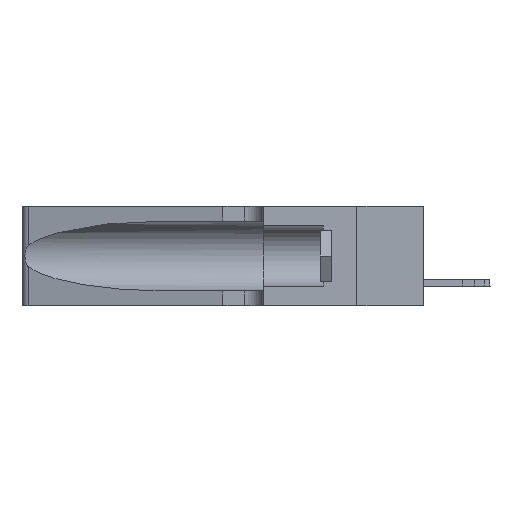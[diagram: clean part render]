
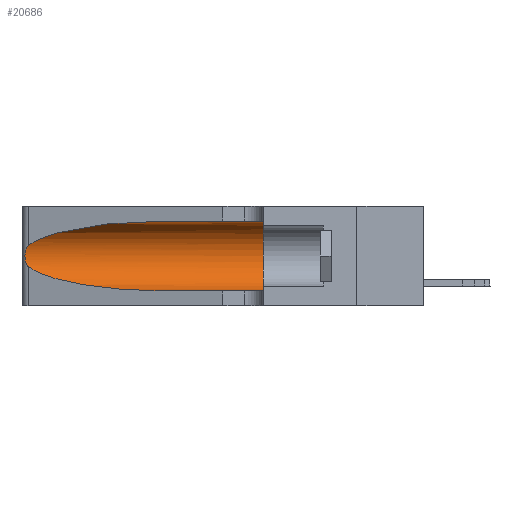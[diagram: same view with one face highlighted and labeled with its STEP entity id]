
A CAD part, left-side view. The second image highlights one B-rep face of the part: STEP entity #20686.
In plain terms, the highlighted cylindrical face has radius 3.308 mm (diameter 6.617 mm), a partial arc.
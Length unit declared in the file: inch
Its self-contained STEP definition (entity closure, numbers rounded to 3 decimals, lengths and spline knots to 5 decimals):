
#1066 = CARTESIAN_POINT ( 'NONE',  ( 0.1305, 1.61858, 0.31525 ) ) ;
#1097 = VERTEX_POINT ( 'NONE', #2380 ) ;
#1640 = CARTESIAN_POINT ( 'NONE',  ( 0.25854, 1.2359, 0.20912 ) ) ;
#2015 = CARTESIAN_POINT ( 'NONE',  ( 0.1305, 0.35, 0.05475 ) ) ;
#2380 = CARTESIAN_POINT ( 'NONE',  ( 0.1305, 0.72297, 0.05475 ) ) ;
#2384 = ORIENTED_EDGE ( 'NONE', *, *, #6230, .T. ) ;
#2564 = CARTESIAN_POINT ( 'NONE',  ( 0.25487, 1.22718, 0.22369 ) ) ;
#2584 = AXIS2_PLACEMENT_3D ( 'NONE', #7743, #18968, #22184 ) ;
#3002 = VERTEX_POINT ( 'NONE', #18890 ) ;
#3477 = CARTESIAN_POINT ( 'NONE',  ( 0.25555, 1.22994, 0.2215 ) ) ;
#3614 = CYLINDRICAL_SURFACE ( 'NONE', #18078, 0.13025 ) ;
#3887 = VECTOR ( 'NONE', #4237, 39.37008 ) ;
#4237 = DIRECTION ( 'NONE',  ( 0., -1., 0. ) ) ;
#4244 =( BOUNDED_CURVE ( )  B_SPLINE_CURVE ( 3, ( #24539, #6105, #8119, #2564 ),
 .UNSPECIFIED., .F., .F. ) 
 B_SPLINE_CURVE_WITH_KNOTS ( ( 4, 4 ),
 ( 1.5708, 2.84003 ),
 .UNSPECIFIED. ) 
 CURVE ( )  GEOMETRIC_REPRESENTATION_ITEM ( )  RATIONAL_B_SPLINE_CURVE ( ( 1., 0.87, 0.87, 1. ) ) 
 REPRESENTATION_ITEM ( '' )  );
#4305 = DIRECTION ( 'NONE',  ( 0., 0., -1. ) ) ;
#4858 = ORIENTED_EDGE ( 'NONE', *, *, #9803, .T. ) ;
#5459 = CARTESIAN_POINT ( 'NONE',  ( 0.2373, 1.15595, 0.08982 ) ) ;
#5894 = EDGE_CURVE ( 'NONE', #9659, #1097, #24818, .T. ) ;
#5911 = ORIENTED_EDGE ( 'NONE', *, *, #20979, .T. ) ;
#6105 = CARTESIAN_POINT ( 'NONE',  ( 0.18966, 0.96281, 0.31525 ) ) ;
#6230 = EDGE_CURVE ( 'NONE', #11029, #9659, #7338, .T. ) ;
#6270 = VECTOR ( 'NONE', #19542, 39.37008 ) ;
#7338 = B_SPLINE_CURVE_WITH_KNOTS ( 'NONE', 3,
 ( #9459, #3477, #17728, #9097, #1640, #19971, #7783, #21850, #9817, #23880, #13670, #7608, #24531, #14824 ),
 .UNSPECIFIED., .F., .F.,
 ( 4, 2, 2, 2, 2, 2, 4 ),
 ( 0., 0.00027, 0.00053, 0.00107, 0.0016, 0.00187, 0.00214 ),
 .UNSPECIFIED. ) ;
#7608 = CARTESIAN_POINT ( 'NONE',  ( 0.25639, 1.23186, 0.15144 ) ) ;
#7743 = CARTESIAN_POINT ( 'NONE',  ( 0.1305, 0.35, 0.185 ) ) ;
#7783 = CARTESIAN_POINT ( 'NONE',  ( 0.26075, 1.23896, 0.19203 ) ) ;
#8119 = CARTESIAN_POINT ( 'NONE',  ( 0.2373, 1.15595, 0.28018 ) ) ;
#9097 = CARTESIAN_POINT ( 'NONE',  ( 0.25787, 1.23484, 0.2124 ) ) ;
#9459 = CARTESIAN_POINT ( 'NONE',  ( 0.25487, 1.22718, 0.22369 ) ) ;
#9659 = VERTEX_POINT ( 'NONE', #11042 ) ;
#9803 = EDGE_CURVE ( 'NONE', #3002, #11029, #4244, .T. ) ;
#9817 = CARTESIAN_POINT ( 'NONE',  ( 0.26017, 1.23833, 0.17102 ) ) ;
#10876 = ORIENTED_EDGE ( 'NONE', *, *, #5894, .T. ) ;
#11019 = LINE ( 'NONE', #1066, #6270 ) ;
#11029 = VERTEX_POINT ( 'NONE', #12679 ) ;
#11042 = CARTESIAN_POINT ( 'NONE',  ( 0.25487, 1.22718, 0.14631 ) ) ;
#11840 = CARTESIAN_POINT ( 'NONE',  ( 0.25487, 1.22718, 0.14631 ) ) ;
#12382 = CIRCLE ( 'NONE', #2584, 0.13025 ) ;
#12679 = CARTESIAN_POINT ( 'NONE',  ( 0.25487, 1.22718, 0.22369 ) ) ;
#12722 = DIRECTION ( 'NONE',  ( 0., -1., 0. ) ) ;
#13479 = EDGE_CURVE ( 'NONE', #24658, #24124, #12382, .T. ) ;
#13670 = CARTESIAN_POINT ( 'NONE',  ( 0.25789, 1.23486, 0.15765 ) ) ;
#13890 = ORIENTED_EDGE ( 'NONE', *, *, #13479, .F. ) ;
#14464 = ORIENTED_EDGE ( 'NONE', *, *, #23758, .F. ) ;
#14824 = CARTESIAN_POINT ( 'NONE',  ( 0.25487, 1.22718, 0.14631 ) ) ;
#15704 = CARTESIAN_POINT ( 'NONE',  ( 0.18966, 0.96281, 0.05475 ) ) ;
#16009 = LINE ( 'NONE', #18688, #3887 ) ;
#16327 = FACE_OUTER_BOUND ( 'NONE', #19758, .T. ) ;
#17728 = CARTESIAN_POINT ( 'NONE',  ( 0.25639, 1.23184, 0.21858 ) ) ;
#18078 = AXIS2_PLACEMENT_3D ( 'NONE', #20910, #12722, #4305 ) ;
#18409 = CARTESIAN_POINT ( 'NONE',  ( 0.1305, 0.35, 0.31525 ) ) ;
#18688 = CARTESIAN_POINT ( 'NONE',  ( 0.1305, 1.61858, 0.05475 ) ) ;
#18890 = CARTESIAN_POINT ( 'NONE',  ( 0.1305, 0.72297, 0.31525 ) ) ;
#18968 = DIRECTION ( 'NONE',  ( 0., 1., 0. ) ) ;
#19542 = DIRECTION ( 'NONE',  ( 0., -1., 0. ) ) ;
#19752 = CARTESIAN_POINT ( 'NONE',  ( 0.1305, 0.72297, 0.05475 ) ) ;
#19758 = EDGE_LOOP ( 'NONE', ( #4858, #2384, #10876, #5911, #13890, #14464 ) ) ;
#19971 = CARTESIAN_POINT ( 'NONE',  ( 0.26018, 1.23835, 0.19895 ) ) ;
#20686 = ADVANCED_FACE ( 'NONE', ( #16327 ), #3614, .F. ) ;
#20910 = CARTESIAN_POINT ( 'NONE',  ( 0.1305, 1.61858, 0.185 ) ) ;
#20979 = EDGE_CURVE ( 'NONE', #1097, #24124, #16009, .T. ) ;
#21850 = CARTESIAN_POINT ( 'NONE',  ( 0.26075, 1.23896, 0.178 ) ) ;
#22184 = DIRECTION ( 'NONE',  ( 0., 0., 1. ) ) ;
#23758 = EDGE_CURVE ( 'NONE', #3002, #24658, #11019, .T. ) ;
#23880 = CARTESIAN_POINT ( 'NONE',  ( 0.25856, 1.23593, 0.16098 ) ) ;
#24124 = VERTEX_POINT ( 'NONE', #2015 ) ;
#24531 = CARTESIAN_POINT ( 'NONE',  ( 0.25555, 1.22993, 0.14849 ) ) ;
#24539 = CARTESIAN_POINT ( 'NONE',  ( 0.1305, 0.72297, 0.31525 ) ) ;
#24658 = VERTEX_POINT ( 'NONE', #18409 ) ;
#24818 =( BOUNDED_CURVE ( )  B_SPLINE_CURVE ( 3, ( #11840, #5459, #15704, #19752 ),
 .UNSPECIFIED., .F., .F. ) 
 B_SPLINE_CURVE_WITH_KNOTS ( ( 4, 4 ),
 ( 3.44316, 4.71239 ),
 .UNSPECIFIED. ) 
 CURVE ( )  GEOMETRIC_REPRESENTATION_ITEM ( )  RATIONAL_B_SPLINE_CURVE ( ( 1., 0.87, 0.87, 1. ) ) 
 REPRESENTATION_ITEM ( '' )  );
